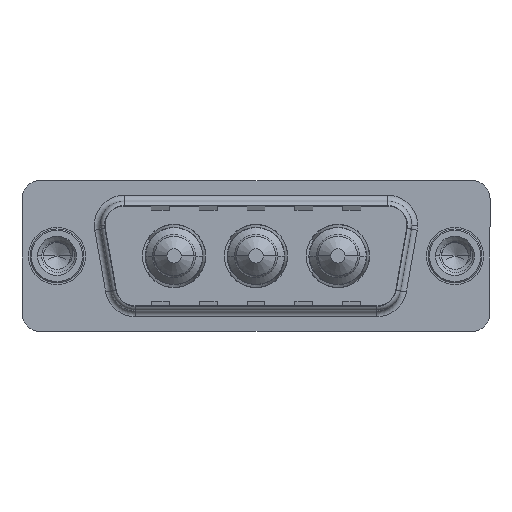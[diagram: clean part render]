
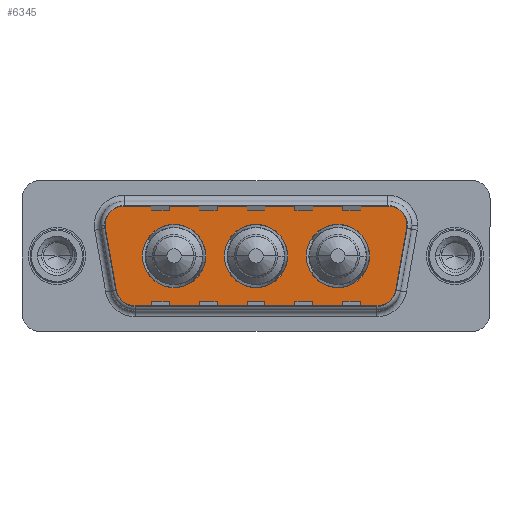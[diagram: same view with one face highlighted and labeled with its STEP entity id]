
A CAD part, top view. The second image highlights one B-rep face of the part: STEP entity #6345.
In plain terms, the highlighted planar face has unit normal (0, 0, 1).
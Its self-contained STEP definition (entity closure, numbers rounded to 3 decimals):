
#192 = EDGE_CURVE ( 'NONE', #3062, #6522, #1058, .T. ) ;
#248 = FACE_BOUND ( 'NONE', #11879, .T. ) ;
#488 = EDGE_CURVE ( 'NONE', #2747, #9525, #1233, .T. ) ;
#510 = CIRCLE ( 'NONE', #12431, 2.65 ) ;
#657 = DIRECTION ( 'NONE',  ( 0., 0., 1. ) ) ;
#982 = DIRECTION ( 'NONE',  ( -1., 0., 0. ) ) ;
#1058 = CIRCLE ( 'NONE', #6998, 2. ) ;
#1124 = CIRCLE ( 'NONE', #10668, 2. ) ;
#1190 = VECTOR ( 'NONE', #9518, 1000. ) ;
#1233 = CIRCLE ( 'NONE', #10141, 2.65 ) ;
#1497 = DIRECTION ( 'NONE',  ( -1., 0., 0. ) ) ;
#1680 = EDGE_CURVE ( 'NONE', #9525, #2747, #10170, .T. ) ;
#1824 = EDGE_LOOP ( 'NONE', ( #6979, #3534 ) ) ;
#1877 = ORIENTED_EDGE ( 'NONE', *, *, #12062, .T. ) ;
#1967 = VERTEX_POINT ( 'NONE', #7874 ) ;
#1974 = AXIS2_PLACEMENT_3D ( 'NONE', #9595, #9542, #9439 ) ;
#1977 = EDGE_CURVE ( 'NONE', #8352, #6692, #3912, .T. ) ;
#2484 = CARTESIAN_POINT ( 'NONE',  ( 29.859, 2.553, 0. ) ) ;
#2539 = ORIENTED_EDGE ( 'NONE', *, *, #3478, .T. ) ;
#2553 = EDGE_CURVE ( 'NONE', #3212, #6394, #510, .T. ) ;
#2619 = CARTESIAN_POINT ( 'NONE',  ( 7.15, 0., 0. ) ) ;
#2747 = VERTEX_POINT ( 'NONE', #9379 ) ;
#2993 = FACE_BOUND ( 'NONE', #4229, .T. ) ;
#3062 = VERTEX_POINT ( 'NONE', #7554 ) ;
#3212 = VERTEX_POINT ( 'NONE', #8981 ) ;
#3216 = DIRECTION ( 'NONE',  ( 0.174, -0.985, 0. ) ) ;
#3221 = AXIS2_PLACEMENT_3D ( 'NONE', #12237, #11261, #1497 ) ;
#3252 = AXIS2_PLACEMENT_3D ( 'NONE', #12260, #657, #11566 ) ;
#3294 = AXIS2_PLACEMENT_3D ( 'NONE', #10321, #4195, #11324 ) ;
#3435 = EDGE_CURVE ( 'NONE', #6522, #10139, #8304, .T. ) ;
#3456 = CARTESIAN_POINT ( 'NONE',  ( 6.434, -4.9, 0. ) ) ;
#3478 = EDGE_CURVE ( 'NONE', #10139, #1967, #5167, .T. ) ;
#3534 = ORIENTED_EDGE ( 'NONE', *, *, #11310, .F. ) ;
#3539 = CARTESIAN_POINT ( 'NONE',  ( 9.8, 0., 0. ) ) ;
#3814 = VERTEX_POINT ( 'NONE', #9206 ) ;
#3822 = VERTEX_POINT ( 'NONE', #9907 ) ;
#3912 = LINE ( 'NONE', #5170, #1190 ) ;
#4108 = EDGE_CURVE ( 'NONE', #11421, #3062, #4187, .T. ) ;
#4187 = LINE ( 'NONE', #3456, #9357 ) ;
#4195 = DIRECTION ( 'NONE',  ( 0., 0., 1. ) ) ;
#4229 = EDGE_LOOP ( 'NONE', ( #9996, #10576 ) ) ;
#4303 = DIRECTION ( 'NONE',  ( 0., 0., 1. ) ) ;
#4390 = CARTESIAN_POINT ( 'NONE',  ( 20.85, 0., 0. ) ) ;
#4440 = CARTESIAN_POINT ( 'NONE',  ( 29.859, 2.553, 0. ) ) ;
#4506 = VECTOR ( 'NONE', #3216, 1000. ) ;
#4515 = ORIENTED_EDGE ( 'NONE', *, *, #4638, .F. ) ;
#4578 = ORIENTED_EDGE ( 'NONE', *, *, #10543, .T. ) ;
#4638 = EDGE_CURVE ( 'NONE', #3814, #3822, #9207, .T. ) ;
#4676 = CIRCLE ( 'NONE', #3294, 2. ) ;
#4956 = DIRECTION ( 'NONE',  ( 1., 0., 0. ) ) ;
#5167 = CIRCLE ( 'NONE', #3221, 2. ) ;
#5170 = CARTESIAN_POINT ( 'NONE',  ( 5.411, 4.9, 0. ) ) ;
#5314 = DIRECTION ( 'NONE',  ( 1., 0., 0. ) ) ;
#5359 = DIRECTION ( 'NONE',  ( 0., 0., 1. ) ) ;
#5380 = ORIENTED_EDGE ( 'NONE', *, *, #11572, .T. ) ;
#5438 = FACE_OUTER_BOUND ( 'NONE', #7595, .T. ) ;
#5513 = VECTOR ( 'NONE', #11621, 1000. ) ;
#5612 = DIRECTION ( 'NONE',  ( 0., 0., 1. ) ) ;
#5833 = DIRECTION ( 'NONE',  ( 1., 0., 0. ) ) ;
#5929 = ORIENTED_EDGE ( 'NONE', *, *, #6832, .T. ) ;
#5978 = AXIS2_PLACEMENT_3D ( 'NONE', #11709, #5612, #12694 ) ;
#6345 = ADVANCED_FACE ( 'NONE', ( #248, #8226, #2993, #5438 ), #9620, .T. ) ;
#6394 = VERTEX_POINT ( 'NONE', #4390 ) ;
#6426 = DIRECTION ( 'NONE',  ( 0., 0., 1. ) ) ;
#6522 = VERTEX_POINT ( 'NONE', #11436 ) ;
#6669 = CARTESIAN_POINT ( 'NONE',  ( 16.65, 0., 0. ) ) ;
#6692 = VERTEX_POINT ( 'NONE', #10848 ) ;
#6801 = CIRCLE ( 'NONE', #5978, 2.65 ) ;
#6832 = EDGE_CURVE ( 'NONE', #6692, #9248, #10202, .T. ) ;
#6856 = ORIENTED_EDGE ( 'NONE', *, *, #192, .T. ) ;
#6905 = AXIS2_PLACEMENT_3D ( 'NONE', #9092, #9050, #8799 ) ;
#6979 = ORIENTED_EDGE ( 'NONE', *, *, #2553, .F. ) ;
#6998 = AXIS2_PLACEMENT_3D ( 'NONE', #7620, #10639, #4956 ) ;
#7183 = DIRECTION ( 'NONE',  ( 0., 0., 1. ) ) ;
#7310 = VERTEX_POINT ( 'NONE', #9880 ) ;
#7554 = CARTESIAN_POINT ( 'NONE',  ( 26.866, -4.9, 0. ) ) ;
#7555 = EDGE_CURVE ( 'NONE', #3822, #3814, #8037, .T. ) ;
#7595 = EDGE_LOOP ( 'NONE', ( #6856, #10374, #2539, #1877, #12152, #5929, #5380, #4578, #11137 ) ) ;
#7620 = CARTESIAN_POINT ( 'NONE',  ( 26.866, -2.9, 0. ) ) ;
#7874 = CARTESIAN_POINT ( 'NONE',  ( 29.889, 2.9, 0. ) ) ;
#7969 = AXIS2_PLACEMENT_3D ( 'NONE', #6669, #6426, #8422 ) ;
#8037 = CIRCLE ( 'NONE', #1974, 2.65 ) ;
#8226 = FACE_BOUND ( 'NONE', #1824, .T. ) ;
#8304 = LINE ( 'NONE', #4440, #5513 ) ;
#8352 = VERTEX_POINT ( 'NONE', #11907 ) ;
#8422 = DIRECTION ( 'NONE',  ( 1., 0., 0. ) ) ;
#8799 = DIRECTION ( 'NONE',  ( 1., 0., 0. ) ) ;
#8981 = CARTESIAN_POINT ( 'NONE',  ( 26.15, 0., 0. ) ) ;
#9007 = CARTESIAN_POINT ( 'NONE',  ( 6.434, -4.9, 0. ) ) ;
#9050 = DIRECTION ( 'NONE',  ( 0., 0., 1. ) ) ;
#9092 = CARTESIAN_POINT ( 'NONE',  ( 5.411, 2.9, 0. ) ) ;
#9206 = CARTESIAN_POINT ( 'NONE',  ( 19.3, 0., 0. ) ) ;
#9207 = CIRCLE ( 'NONE', #7969, 2.65 ) ;
#9248 = VERTEX_POINT ( 'NONE', #12418 ) ;
#9301 = DIRECTION ( 'NONE',  ( 0., 0., 1. ) ) ;
#9315 = DIRECTION ( 'NONE',  ( 1., 0., 0. ) ) ;
#9357 = VECTOR ( 'NONE', #5833, 1000. ) ;
#9358 = LINE ( 'NONE', #9398, #4506 ) ;
#9379 = CARTESIAN_POINT ( 'NONE',  ( 12.45, 0., 0. ) ) ;
#9398 = CARTESIAN_POINT ( 'NONE',  ( 3.441, 2.553, 0. ) ) ;
#9439 = DIRECTION ( 'NONE',  ( 1., 0., 0. ) ) ;
#9518 = DIRECTION ( 'NONE',  ( -1., 0., 0. ) ) ;
#9525 = VERTEX_POINT ( 'NONE', #2619 ) ;
#9542 = DIRECTION ( 'NONE',  ( 0., 0., 1. ) ) ;
#9595 = CARTESIAN_POINT ( 'NONE',  ( 16.65, 0., 0. ) ) ;
#9620 = PLANE ( 'NONE',  #3252 ) ;
#9880 = CARTESIAN_POINT ( 'NONE',  ( 4.464, -3.247, 0. ) ) ;
#9907 = CARTESIAN_POINT ( 'NONE',  ( 14., 0., 0. ) ) ;
#9996 = ORIENTED_EDGE ( 'NONE', *, *, #488, .F. ) ;
#10139 = VERTEX_POINT ( 'NONE', #2484 ) ;
#10141 = AXIS2_PLACEMENT_3D ( 'NONE', #3539, #4303, #13182 ) ;
#10170 = CIRCLE ( 'NONE', #10480, 2.65 ) ;
#10202 = CIRCLE ( 'NONE', #6905, 2. ) ;
#10321 = CARTESIAN_POINT ( 'NONE',  ( 6.434, -2.9, 0. ) ) ;
#10374 = ORIENTED_EDGE ( 'NONE', *, *, #3435, .T. ) ;
#10480 = AXIS2_PLACEMENT_3D ( 'NONE', #10596, #9301, #9315 ) ;
#10543 = EDGE_CURVE ( 'NONE', #7310, #11421, #4676, .T. ) ;
#10576 = ORIENTED_EDGE ( 'NONE', *, *, #1680, .F. ) ;
#10596 = CARTESIAN_POINT ( 'NONE',  ( 9.8, 0., 0. ) ) ;
#10639 = DIRECTION ( 'NONE',  ( 0., 0., 1. ) ) ;
#10668 = AXIS2_PLACEMENT_3D ( 'NONE', #13184, #7183, #982 ) ;
#10848 = CARTESIAN_POINT ( 'NONE',  ( 5.411, 4.9, 0. ) ) ;
#10987 = ORIENTED_EDGE ( 'NONE', *, *, #7555, .F. ) ;
#11137 = ORIENTED_EDGE ( 'NONE', *, *, #4108, .T. ) ;
#11261 = DIRECTION ( 'NONE',  ( 0., 0., 1. ) ) ;
#11310 = EDGE_CURVE ( 'NONE', #6394, #3212, #6801, .T. ) ;
#11324 = DIRECTION ( 'NONE',  ( -1., 0., 0. ) ) ;
#11421 = VERTEX_POINT ( 'NONE', #9007 ) ;
#11436 = CARTESIAN_POINT ( 'NONE',  ( 28.836, -3.247, 0. ) ) ;
#11566 = DIRECTION ( 'NONE',  ( 1., 0., 0. ) ) ;
#11572 = EDGE_CURVE ( 'NONE', #9248, #7310, #9358, .T. ) ;
#11621 = DIRECTION ( 'NONE',  ( 0.174, 0.985, 0. ) ) ;
#11709 = CARTESIAN_POINT ( 'NONE',  ( 23.5, 0., 0. ) ) ;
#11879 = EDGE_LOOP ( 'NONE', ( #4515, #10987 ) ) ;
#11907 = CARTESIAN_POINT ( 'NONE',  ( 27.889, 4.9, 0. ) ) ;
#12062 = EDGE_CURVE ( 'NONE', #1967, #8352, #1124, .T. ) ;
#12152 = ORIENTED_EDGE ( 'NONE', *, *, #1977, .T. ) ;
#12237 = CARTESIAN_POINT ( 'NONE',  ( 27.889, 2.9, 0. ) ) ;
#12260 = CARTESIAN_POINT ( 'NONE',  ( 26.866, -2.9, 0. ) ) ;
#12418 = CARTESIAN_POINT ( 'NONE',  ( 3.441, 2.553, 0. ) ) ;
#12431 = AXIS2_PLACEMENT_3D ( 'NONE', #12559, #5359, #5314 ) ;
#12559 = CARTESIAN_POINT ( 'NONE',  ( 23.5, 0., 0. ) ) ;
#12694 = DIRECTION ( 'NONE',  ( 1., 0., 0. ) ) ;
#13182 = DIRECTION ( 'NONE',  ( 1., 0., 0. ) ) ;
#13184 = CARTESIAN_POINT ( 'NONE',  ( 27.889, 2.9, 0. ) ) ;
